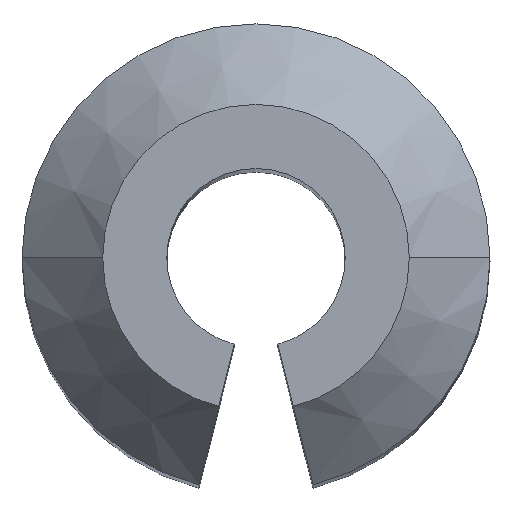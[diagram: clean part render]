
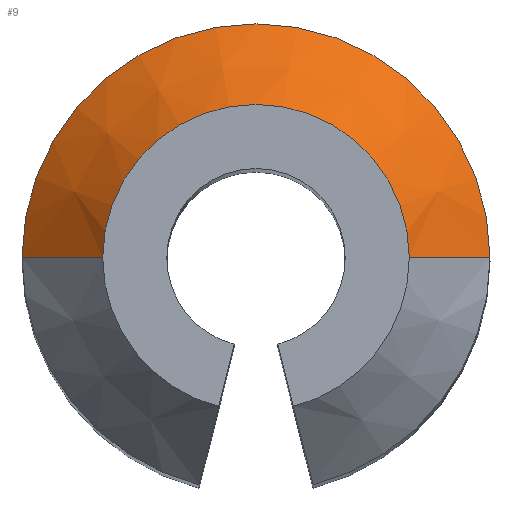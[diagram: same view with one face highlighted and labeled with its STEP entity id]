
A CAD part, top view. The second image highlights one B-rep face of the part: STEP entity #9.
In plain terms, the highlighted conical face has half-angle 45 degrees and reference radius 1.041 mm.
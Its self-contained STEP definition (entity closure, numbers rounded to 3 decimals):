
#9 = ADVANCED_FACE ( 'NONE', ( #508 ), #498, .T. ) ;
#43 = ORIENTED_EDGE ( 'NONE', *, *, #397, .T. ) ;
#63 = VERTEX_POINT ( 'NONE', #373 ) ;
#98 = EDGE_LOOP ( 'NONE', ( #130, #43, #100, #242 ) ) ;
#100 = ORIENTED_EDGE ( 'NONE', *, *, #412, .F. ) ;
#108 = DIRECTION ( 'NONE',  ( 0., 0., -1. ) ) ;
#118 = CIRCLE ( 'NONE', #385, 1.041 ) ;
#127 = VERTEX_POINT ( 'NONE', #354 ) ;
#130 = ORIENTED_EDGE ( 'NONE', *, *, #393, .T. ) ;
#145 = CIRCLE ( 'NONE', #333, 0.682 ) ;
#183 = VERTEX_POINT ( 'NONE', #349 ) ;
#184 = VERTEX_POINT ( 'NONE', #352 ) ;
#240 = DIRECTION ( 'NONE',  ( 1., 0., 0. ) ) ;
#242 = ORIENTED_EDGE ( 'NONE', *, *, #400, .F. ) ;
#243 = DIRECTION ( 'NONE',  ( 0., 0., -1. ) ) ;
#244 = CARTESIAN_POINT ( 'NONE',  ( 0., 0., -0.359 ) ) ;
#281 = DIRECTION ( 'NONE',  ( -0.707, 0., -0.707 ) ) ;
#284 = DIRECTION ( 'NONE',  ( -1., 0., 0. ) ) ;
#285 = DIRECTION ( 'NONE',  ( 0., 0., -1. ) ) ;
#286 = CARTESIAN_POINT ( 'NONE',  ( 0., 0., 0. ) ) ;
#287 = CARTESIAN_POINT ( 'NONE',  ( 1.041, 0., -0.359 ) ) ;
#291 = CARTESIAN_POINT ( 'NONE',  ( -1.041, 0., -0.359 ) ) ;
#298 = DIRECTION ( 'NONE',  ( 0.707, 0., -0.707 ) ) ;
#330 = LINE ( 'NONE', #291, #390 ) ;
#333 = AXIS2_PLACEMENT_3D ( 'NONE', #286, #285, #284 ) ;
#349 = CARTESIAN_POINT ( 'NONE',  ( 1.041, 0., -0.359 ) ) ;
#352 = CARTESIAN_POINT ( 'NONE',  ( -1.041, 0., -0.359 ) ) ;
#354 = CARTESIAN_POINT ( 'NONE',  ( -0.682, 0., 0. ) ) ;
#369 = LINE ( 'NONE', #287, #509 ) ;
#373 = CARTESIAN_POINT ( 'NONE',  ( 0.682, 0., 0. ) ) ;
#385 = AXIS2_PLACEMENT_3D ( 'NONE', #244, #243, #240 ) ;
#390 = VECTOR ( 'NONE', #281, 1000. ) ;
#393 = EDGE_CURVE ( 'NONE', #127, #63, #145, .T. ) ;
#397 = EDGE_CURVE ( 'NONE', #63, #183, #369, .T. ) ;
#400 = EDGE_CURVE ( 'NONE', #127, #184, #330, .T. ) ;
#412 = EDGE_CURVE ( 'NONE', #184, #183, #118, .T. ) ;
#423 = AXIS2_PLACEMENT_3D ( 'NONE', #510, #108, #499 ) ;
#498 = CONICAL_SURFACE ( 'NONE', #423, 1.041, 0.785 ) ;
#499 = DIRECTION ( 'NONE',  ( -1., 0., 0. ) ) ;
#508 = FACE_OUTER_BOUND ( 'NONE', #98, .T. ) ;
#509 = VECTOR ( 'NONE', #298, 1000. ) ;
#510 = CARTESIAN_POINT ( 'NONE',  ( 0., 0., -0.359 ) ) ;
